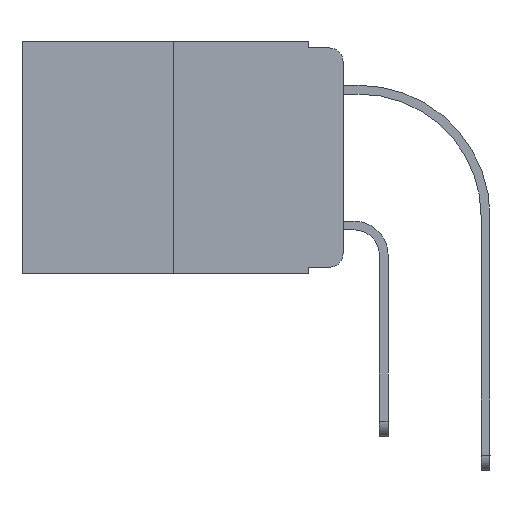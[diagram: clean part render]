
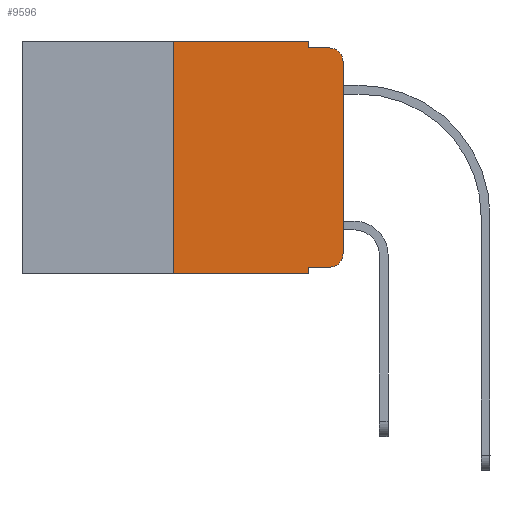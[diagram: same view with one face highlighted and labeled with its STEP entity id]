
A CAD part, left-side view. The second image highlights one B-rep face of the part: STEP entity #9596.
In plain terms, the highlighted planar face has unit normal (-1, 0, 0).
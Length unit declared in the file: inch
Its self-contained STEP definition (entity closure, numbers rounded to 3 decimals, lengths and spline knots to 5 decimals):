
#536 = CARTESIAN_POINT ( 'NONE',  ( 0., 0.473, -0.343 ) ) ;
#825 = LINE ( 'NONE', #536, #19657 ) ;
#1084 = EDGE_CURVE ( 'NONE', #9801, #1440, #16753, .T. ) ;
#1291 = DIRECTION ( 'NONE',  ( 0., 0., -1. ) ) ;
#1414 = DIRECTION ( 'NONE',  ( -1., 0., 0. ) ) ;
#1440 = VERTEX_POINT ( 'NONE', #7012 ) ;
#1441 = CARTESIAN_POINT ( 'NONE',  ( 0., 0.473, 0. ) ) ;
#1532 = LINE ( 'NONE', #18816, #22637 ) ;
#2186 = ORIENTED_EDGE ( 'NONE', *, *, #19894, .T. ) ;
#2558 = EDGE_CURVE ( 'NONE', #9363, #15884, #14916, .T. ) ;
#2903 = CARTESIAN_POINT ( 'NONE',  ( 0., 0.25, 0. ) ) ;
#3277 = VERTEX_POINT ( 'NONE', #5287 ) ;
#3460 = AXIS2_PLACEMENT_3D ( 'NONE', #22309, #12307, #16375 ) ;
#3738 = AXIS2_PLACEMENT_3D ( 'NONE', #18375, #23131, #25099 ) ;
#4066 = DIRECTION ( 'NONE',  ( 0., 0., 1. ) ) ;
#4095 = CARTESIAN_POINT ( 'NONE',  ( 0., 0.051, 0. ) ) ;
#4416 = VERTEX_POINT ( 'NONE', #19362 ) ;
#4464 = EDGE_CURVE ( 'NONE', #16629, #11295, #825, .T. ) ;
#4578 = CARTESIAN_POINT ( 'NONE',  ( 0., 0., -0.03 ) ) ;
#5287 = CARTESIAN_POINT ( 'NONE',  ( 0., 0., -0.313 ) ) ;
#5790 = CARTESIAN_POINT ( 'NONE',  ( 0., 0.051, -0.333 ) ) ;
#6898 = CARTESIAN_POINT ( 'NONE',  ( 0., 0.051, -0.01 ) ) ;
#7012 = CARTESIAN_POINT ( 'NONE',  ( 0., 0.02, -0.01 ) ) ;
#7482 = DIRECTION ( 'NONE',  ( 0., -1., 0. ) ) ;
#8297 = EDGE_LOOP ( 'NONE', ( #2186, #27342, #24077, #9623, #21757, #14978, #20925, #17848, #25833, #21003 ) ) ;
#8370 = VECTOR ( 'NONE', #20248, 39.37008 ) ;
#8758 = LINE ( 'NONE', #14660, #20020 ) ;
#8850 = CIRCLE ( 'NONE', #3460, 0.02 ) ;
#9363 = VERTEX_POINT ( 'NONE', #19367 ) ;
#9596 = ADVANCED_FACE ( 'NONE', ( #20598 ), #18793, .F. ) ;
#9623 = ORIENTED_EDGE ( 'NONE', *, *, #2558, .F. ) ;
#9758 = LINE ( 'NONE', #1441, #8370 ) ;
#9801 = VERTEX_POINT ( 'NONE', #4578 ) ;
#9863 = CARTESIAN_POINT ( 'NONE',  ( 0., 0.02, -0.03 ) ) ;
#11295 = VERTEX_POINT ( 'NONE', #13586 ) ;
#11960 = VECTOR ( 'NONE', #21933, 39.37008 ) ;
#11969 = EDGE_CURVE ( 'NONE', #26112, #4416, #16619, .T. ) ;
#12192 = EDGE_CURVE ( 'NONE', #15884, #1440, #26143, .T. ) ;
#12307 = DIRECTION ( 'NONE',  ( -1., 0., 0. ) ) ;
#12802 = EDGE_CURVE ( 'NONE', #4416, #3277, #8850, .T. ) ;
#13586 = CARTESIAN_POINT ( 'NONE',  ( 0., 0.051, -0.343 ) ) ;
#14660 = CARTESIAN_POINT ( 'NONE',  ( 0., 0.051, 0. ) ) ;
#14845 = LINE ( 'NONE', #23393, #25326 ) ;
#14916 = LINE ( 'NONE', #4095, #15063 ) ;
#14978 = ORIENTED_EDGE ( 'NONE', *, *, #20610, .F. ) ;
#15058 = DIRECTION ( 'NONE',  ( 0., 0., -1. ) ) ;
#15063 = VECTOR ( 'NONE', #15058, 39.37008 ) ;
#15884 = VERTEX_POINT ( 'NONE', #19167 ) ;
#16375 = DIRECTION ( 'NONE',  ( 0., 0., -1. ) ) ;
#16619 = LINE ( 'NONE', #5790, #18653 ) ;
#16629 = VERTEX_POINT ( 'NONE', #22692 ) ;
#16753 = CIRCLE ( 'NONE', #26166, 0.02 ) ;
#17848 = ORIENTED_EDGE ( 'NONE', *, *, #24242, .F. ) ;
#18375 = CARTESIAN_POINT ( 'NONE',  ( 0., 0.473, 0. ) ) ;
#18653 = VECTOR ( 'NONE', #7482, 39.37008 ) ;
#18793 = PLANE ( 'NONE',  #3738 ) ;
#18816 = CARTESIAN_POINT ( 'NONE',  ( 0., 0.25, 0. ) ) ;
#19167 = CARTESIAN_POINT ( 'NONE',  ( 0., 0.051, -0.01 ) ) ;
#19362 = CARTESIAN_POINT ( 'NONE',  ( 0., 0.02, -0.333 ) ) ;
#19367 = CARTESIAN_POINT ( 'NONE',  ( 0., 0.051, 0. ) ) ;
#19657 = VECTOR ( 'NONE', #23730, 39.37008 ) ;
#19894 = EDGE_CURVE ( 'NONE', #3277, #9801, #14845, .T. ) ;
#20020 = VECTOR ( 'NONE', #23217, 39.37008 ) ;
#20245 = CARTESIAN_POINT ( 'NONE',  ( 0., 0.051, -0.333 ) ) ;
#20248 = DIRECTION ( 'NONE',  ( 0., -1., 0. ) ) ;
#20598 = FACE_OUTER_BOUND ( 'NONE', #8297, .T. ) ;
#20610 = EDGE_CURVE ( 'NONE', #16629, #25421, #1532, .T. ) ;
#20925 = ORIENTED_EDGE ( 'NONE', *, *, #4464, .T. ) ;
#21003 = ORIENTED_EDGE ( 'NONE', *, *, #12802, .T. ) ;
#21284 = DIRECTION ( 'NONE',  ( 0., 0., 1. ) ) ;
#21757 = ORIENTED_EDGE ( 'NONE', *, *, #24055, .F. ) ;
#21933 = DIRECTION ( 'NONE',  ( 0., -1., 0. ) ) ;
#22309 = CARTESIAN_POINT ( 'NONE',  ( 0., 0.02, -0.313 ) ) ;
#22637 = VECTOR ( 'NONE', #4066, 39.37008 ) ;
#22692 = CARTESIAN_POINT ( 'NONE',  ( 0., 0.25, -0.343 ) ) ;
#23131 = DIRECTION ( 'NONE',  ( 1., 0., 0. ) ) ;
#23217 = DIRECTION ( 'NONE',  ( 0., 0., -1. ) ) ;
#23393 = CARTESIAN_POINT ( 'NONE',  ( 0., 0., 0. ) ) ;
#23730 = DIRECTION ( 'NONE',  ( 0., -1., 0. ) ) ;
#24055 = EDGE_CURVE ( 'NONE', #25421, #9363, #9758, .T. ) ;
#24077 = ORIENTED_EDGE ( 'NONE', *, *, #12192, .F. ) ;
#24242 = EDGE_CURVE ( 'NONE', #26112, #11295, #8758, .T. ) ;
#25099 = DIRECTION ( 'NONE',  ( 0., 0., -1. ) ) ;
#25326 = VECTOR ( 'NONE', #21284, 39.37008 ) ;
#25421 = VERTEX_POINT ( 'NONE', #2903 ) ;
#25833 = ORIENTED_EDGE ( 'NONE', *, *, #11969, .T. ) ;
#26112 = VERTEX_POINT ( 'NONE', #20245 ) ;
#26143 = LINE ( 'NONE', #6898, #11960 ) ;
#26166 = AXIS2_PLACEMENT_3D ( 'NONE', #9863, #1414, #1291 ) ;
#27342 = ORIENTED_EDGE ( 'NONE', *, *, #1084, .T. ) ;
